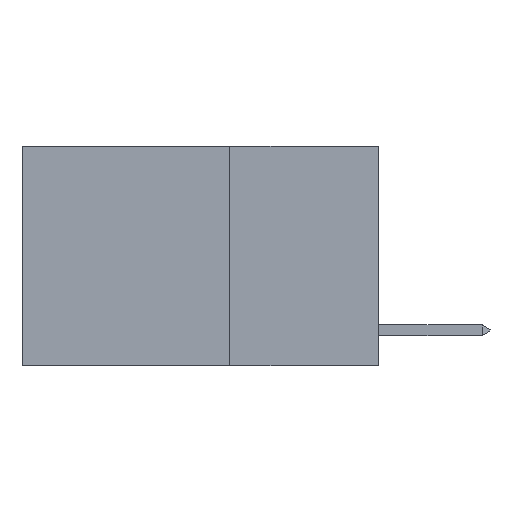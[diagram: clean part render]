
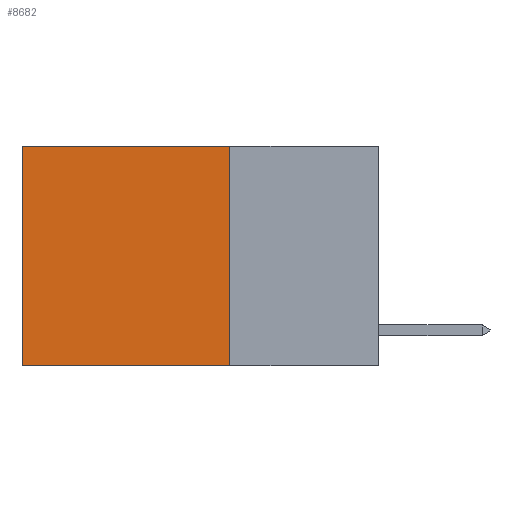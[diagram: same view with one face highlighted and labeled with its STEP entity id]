
A CAD part, left-side view. The second image highlights one B-rep face of the part: STEP entity #8682.
In plain terms, the highlighted planar face has unit normal (-1, 0, 0).
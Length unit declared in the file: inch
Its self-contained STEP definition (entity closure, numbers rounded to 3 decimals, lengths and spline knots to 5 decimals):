
#25 = EDGE_CURVE ( 'NONE', #595, #6363, #3173, .T. ) ;
#434 = CARTESIAN_POINT ( 'NONE',  ( 0.2625, 0.25, -0.37 ) ) ;
#559 = VERTEX_POINT ( 'NONE', #4873 ) ;
#595 = VERTEX_POINT ( 'NONE', #3175 ) ;
#752 = VECTOR ( 'NONE', #8060, 39.37008 ) ;
#846 = VECTOR ( 'NONE', #7869, 39.37008 ) ;
#1081 = CARTESIAN_POINT ( 'NONE',  ( 0.2625, 0.25, 0. ) ) ;
#1164 = DIRECTION ( 'NONE',  ( 0., 0., -1. ) ) ;
#1702 = DIRECTION ( 'NONE',  ( 0., 0., -1. ) ) ;
#1752 = DIRECTION ( 'NONE',  ( 1., 0., 0. ) ) ;
#2428 = VECTOR ( 'NONE', #1702, 39.37008 ) ;
#2442 = CARTESIAN_POINT ( 'NONE',  ( 0.2625, 0.25, 0. ) ) ;
#2632 = LINE ( 'NONE', #4524, #752 ) ;
#2817 = DIRECTION ( 'NONE',  ( 0., 1., 0. ) ) ;
#3049 = VECTOR ( 'NONE', #2817, 39.37008 ) ;
#3055 = PLANE ( 'NONE',  #4649 ) ;
#3173 = LINE ( 'NONE', #1081, #846 ) ;
#3175 = CARTESIAN_POINT ( 'NONE',  ( 0.2625, 0.25, 0. ) ) ;
#3704 = VERTEX_POINT ( 'NONE', #7755 ) ;
#4524 = CARTESIAN_POINT ( 'NONE',  ( 0.2625, 0.25, -0.37 ) ) ;
#4649 = AXIS2_PLACEMENT_3D ( 'NONE', #2442, #1752, #1164 ) ;
#4873 = CARTESIAN_POINT ( 'NONE',  ( 0.2625, 0.6, -0.37 ) ) ;
#4999 = LINE ( 'NONE', #7727, #2428 ) ;
#5598 = EDGE_LOOP ( 'NONE', ( #7049, #6632, #7430, #7313 ) ) ;
#5637 = EDGE_CURVE ( 'NONE', #595, #3704, #8172, .T. ) ;
#6208 = CARTESIAN_POINT ( 'NONE',  ( 0.2625, 0.25, 0. ) ) ;
#6363 = VERTEX_POINT ( 'NONE', #434 ) ;
#6632 = ORIENTED_EDGE ( 'NONE', *, *, #8113, .F. ) ;
#7049 = ORIENTED_EDGE ( 'NONE', *, *, #7753, .T. ) ;
#7209 = FACE_OUTER_BOUND ( 'NONE', #5598, .T. ) ;
#7313 = ORIENTED_EDGE ( 'NONE', *, *, #5637, .T. ) ;
#7430 = ORIENTED_EDGE ( 'NONE', *, *, #25, .F. ) ;
#7727 = CARTESIAN_POINT ( 'NONE',  ( 0.2625, 0.6, 0. ) ) ;
#7753 = EDGE_CURVE ( 'NONE', #3704, #559, #4999, .T. ) ;
#7755 = CARTESIAN_POINT ( 'NONE',  ( 0.2625, 0.6, 0. ) ) ;
#7869 = DIRECTION ( 'NONE',  ( 0., 0., -1. ) ) ;
#8060 = DIRECTION ( 'NONE',  ( 0., 1., 0. ) ) ;
#8113 = EDGE_CURVE ( 'NONE', #6363, #559, #2632, .T. ) ;
#8172 = LINE ( 'NONE', #6208, #3049 ) ;
#8682 = ADVANCED_FACE ( 'NONE', ( #7209 ), #3055, .F. ) ;
